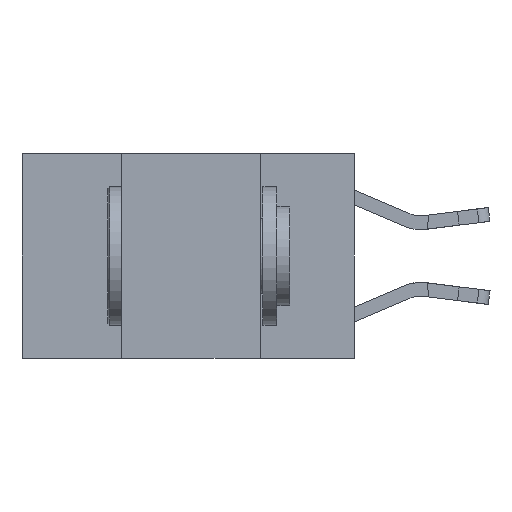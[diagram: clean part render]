
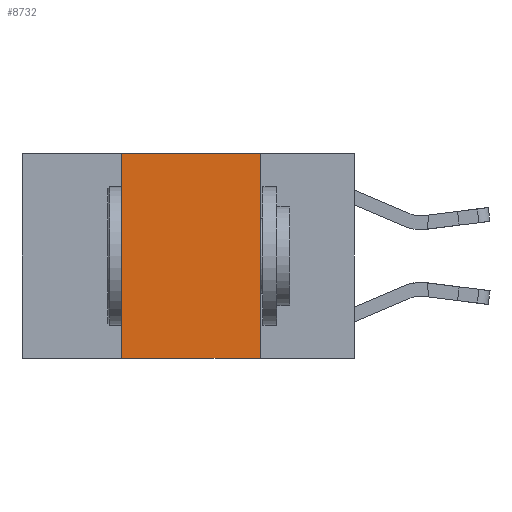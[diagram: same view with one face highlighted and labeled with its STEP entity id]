
A CAD part, left-side view. The second image highlights one B-rep face of the part: STEP entity #8732.
In plain terms, the highlighted planar face has unit normal (-1, 0, 0).
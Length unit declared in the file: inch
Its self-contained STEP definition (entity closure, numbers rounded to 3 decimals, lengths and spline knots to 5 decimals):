
#234 = ORIENTED_EDGE ( 'NONE', *, *, #474, .F. ) ;
#443 = CARTESIAN_POINT ( 'NONE',  ( 0., 0.17, -0.37 ) ) ;
#471 = DIRECTION ( 'NONE',  ( 0., -1., 0. ) ) ;
#474 = EDGE_CURVE ( 'NONE', #7759, #16260, #7976, .T. ) ;
#750 = EDGE_CURVE ( 'NONE', #8861, #4302, #14347, .T. ) ;
#976 = ORIENTED_EDGE ( 'NONE', *, *, #16989, .T. ) ;
#1168 = VECTOR ( 'NONE', #10279, 39.37008 ) ;
#2724 = CARTESIAN_POINT ( 'NONE',  ( 0., 0.6, -0.37 ) ) ;
#2847 = ORIENTED_EDGE ( 'NONE', *, *, #17671, .F. ) ;
#4302 = VERTEX_POINT ( 'NONE', #16206 ) ;
#6077 = LINE ( 'NONE', #9097, #8136 ) ;
#6717 = CARTESIAN_POINT ( 'NONE',  ( 0., 0.17, 0. ) ) ;
#6843 = PLANE ( 'NONE',  #16936 ) ;
#7173 = LINE ( 'NONE', #2724, #12435 ) ;
#7355 = ORIENTED_EDGE ( 'NONE', *, *, #750, .F. ) ;
#7759 = VERTEX_POINT ( 'NONE', #11880 ) ;
#7976 = LINE ( 'NONE', #6717, #19109 ) ;
#8136 = VECTOR ( 'NONE', #471, 39.37008 ) ;
#8732 = ADVANCED_FACE ( 'NONE', ( #15648 ), #6843, .F. ) ;
#8861 = VERTEX_POINT ( 'NONE', #12009 ) ;
#9097 = CARTESIAN_POINT ( 'NONE',  ( 0., 0.6, 0. ) ) ;
#10279 = DIRECTION ( 'NONE',  ( 0., 0., 1. ) ) ;
#11086 = DIRECTION ( 'NONE',  ( 0., 0., -1. ) ) ;
#11880 = CARTESIAN_POINT ( 'NONE',  ( 0., 0.17, 0. ) ) ;
#12009 = CARTESIAN_POINT ( 'NONE',  ( 0., 0.42, -0.37 ) ) ;
#12399 = DIRECTION ( 'NONE',  ( 0., 0., -1. ) ) ;
#12435 = VECTOR ( 'NONE', #13063, 39.37008 ) ;
#12633 = CARTESIAN_POINT ( 'NONE',  ( 0., 0.6, 0. ) ) ;
#13063 = DIRECTION ( 'NONE',  ( 0., -1., 0. ) ) ;
#14347 = LINE ( 'NONE', #17665, #1168 ) ;
#14561 = EDGE_LOOP ( 'NONE', ( #234, #2847, #7355, #976 ) ) ;
#15648 = FACE_OUTER_BOUND ( 'NONE', #14561, .T. ) ;
#16206 = CARTESIAN_POINT ( 'NONE',  ( 0., 0.42, 0. ) ) ;
#16260 = VERTEX_POINT ( 'NONE', #443 ) ;
#16936 = AXIS2_PLACEMENT_3D ( 'NONE', #12633, #18576, #11086 ) ;
#16989 = EDGE_CURVE ( 'NONE', #8861, #16260, #7173, .T. ) ;
#17665 = CARTESIAN_POINT ( 'NONE',  ( 0., 0.42, 0. ) ) ;
#17671 = EDGE_CURVE ( 'NONE', #4302, #7759, #6077, .T. ) ;
#18576 = DIRECTION ( 'NONE',  ( 1., 0., 0. ) ) ;
#19109 = VECTOR ( 'NONE', #12399, 39.37008 ) ;
